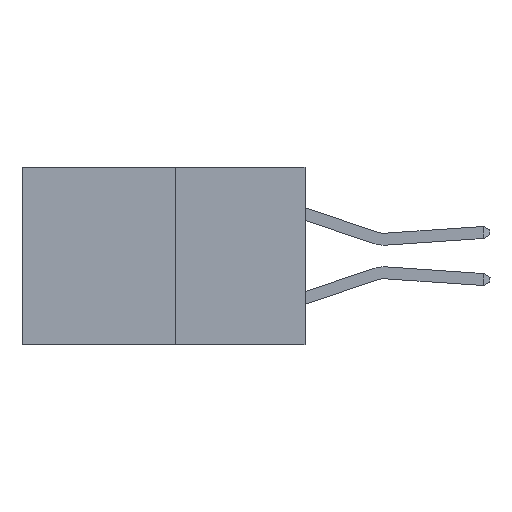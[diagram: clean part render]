
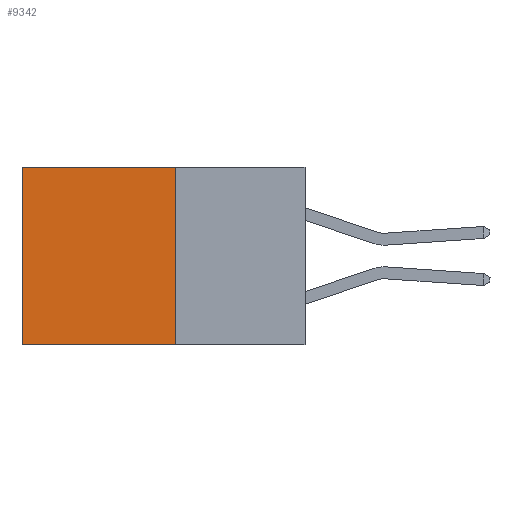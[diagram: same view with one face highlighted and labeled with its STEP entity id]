
A CAD part, left-side view. The second image highlights one B-rep face of the part: STEP entity #9342.
In plain terms, the highlighted planar face has unit normal (-1, 0, 0).
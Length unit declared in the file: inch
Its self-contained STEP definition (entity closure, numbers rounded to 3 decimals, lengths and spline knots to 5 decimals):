
#228 = EDGE_CURVE ( 'NONE', #2989, #21684, #19197, .T. ) ;
#235 = DIRECTION ( 'NONE',  ( 0., 0., -1. ) ) ;
#681 = ORIENTED_EDGE ( 'NONE', *, *, #10459, .T. ) ;
#1986 = ORIENTED_EDGE ( 'NONE', *, *, #21848, .F. ) ;
#2372 = VERTEX_POINT ( 'NONE', #12582 ) ;
#2703 = VECTOR ( 'NONE', #6124, 39.37008 ) ;
#2964 = CARTESIAN_POINT ( 'NONE',  ( 0.277, 0.27, -0.37 ) ) ;
#2989 = VERTEX_POINT ( 'NONE', #21363 ) ;
#3115 = CARTESIAN_POINT ( 'NONE',  ( 0.277, 0.27, -0.37 ) ) ;
#3730 = CARTESIAN_POINT ( 'NONE',  ( 0.277, 0.59, -0.37 ) ) ;
#3979 = AXIS2_PLACEMENT_3D ( 'NONE', #7795, #7371, #7369 ) ;
#4175 = CARTESIAN_POINT ( 'NONE',  ( 0.277, 0.59, 0. ) ) ;
#5927 = LINE ( 'NONE', #3730, #14051 ) ;
#6124 = DIRECTION ( 'NONE',  ( 0., 0., -1. ) ) ;
#7369 = DIRECTION ( 'NONE',  ( 0., 0., -1. ) ) ;
#7371 = DIRECTION ( 'NONE',  ( 1., 0., 0. ) ) ;
#7472 = PLANE ( 'NONE',  #3979 ) ;
#7795 = CARTESIAN_POINT ( 'NONE',  ( 0.277, 0.27, -0.37 ) ) ;
#9226 = FACE_OUTER_BOUND ( 'NONE', #17080, .T. ) ;
#9342 = ADVANCED_FACE ( 'NONE', ( #9226 ), #7472, .F. ) ;
#10459 = EDGE_CURVE ( 'NONE', #21684, #2372, #5927, .T. ) ;
#11512 = DIRECTION ( 'NONE',  ( 0., 1., 0. ) ) ;
#11829 = LINE ( 'NONE', #14745, #2703 ) ;
#11847 = LINE ( 'NONE', #2964, #16508 ) ;
#12582 = CARTESIAN_POINT ( 'NONE',  ( 0.277, 0.59, -0.37 ) ) ;
#13834 = VERTEX_POINT ( 'NONE', #3115 ) ;
#14051 = VECTOR ( 'NONE', #235, 39.37008 ) ;
#14509 = VECTOR ( 'NONE', #21705, 39.37008 ) ;
#14745 = CARTESIAN_POINT ( 'NONE',  ( 0.277, 0.27, -0.37 ) ) ;
#15098 = ORIENTED_EDGE ( 'NONE', *, *, #228, .T. ) ;
#16508 = VECTOR ( 'NONE', #11512, 39.37008 ) ;
#17080 = EDGE_LOOP ( 'NONE', ( #681, #1986, #20577, #15098 ) ) ;
#17665 = CARTESIAN_POINT ( 'NONE',  ( 0.277, 0.27, 0. ) ) ;
#19197 = LINE ( 'NONE', #17665, #14509 ) ;
#19237 = EDGE_CURVE ( 'NONE', #2989, #13834, #11829, .T. ) ;
#20577 = ORIENTED_EDGE ( 'NONE', *, *, #19237, .F. ) ;
#21363 = CARTESIAN_POINT ( 'NONE',  ( 0.277, 0.27, 0. ) ) ;
#21684 = VERTEX_POINT ( 'NONE', #4175 ) ;
#21705 = DIRECTION ( 'NONE',  ( 0., 1., 0. ) ) ;
#21848 = EDGE_CURVE ( 'NONE', #13834, #2372, #11847, .T. ) ;
